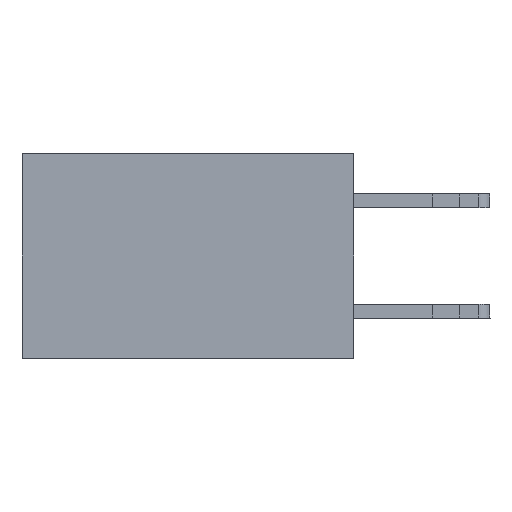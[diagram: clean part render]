
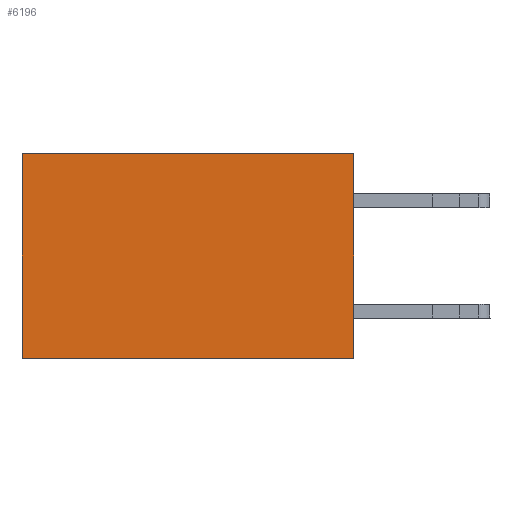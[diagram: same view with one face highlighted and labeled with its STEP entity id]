
A CAD part, left-side view. The second image highlights one B-rep face of the part: STEP entity #6196.
In plain terms, the highlighted planar face has unit normal (-1, 0, 0).
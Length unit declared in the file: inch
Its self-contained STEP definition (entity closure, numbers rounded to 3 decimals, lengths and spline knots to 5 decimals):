
#763 = DIRECTION ( 'NONE',  ( 0., 0., -1. ) ) ;
#1288 = VECTOR ( 'NONE', #11786, 39.37008 ) ;
#1577 = CARTESIAN_POINT ( 'NONE',  ( 0.2875, 0.6, -0.37 ) ) ;
#2237 = CARTESIAN_POINT ( 'NONE',  ( 0.2875, 0., -0.37 ) ) ;
#2305 = VECTOR ( 'NONE', #763, 39.37008 ) ;
#2589 = CARTESIAN_POINT ( 'NONE',  ( 0.2875, 0., 0. ) ) ;
#3010 = LINE ( 'NONE', #9871, #11471 ) ;
#3818 = EDGE_CURVE ( 'NONE', #21166, #11172, #21135, .T. ) ;
#5787 = ORIENTED_EDGE ( 'NONE', *, *, #3818, .T. ) ;
#6196 = ADVANCED_FACE ( 'NONE', ( #18928 ), #8611, .F. ) ;
#6915 = LINE ( 'NONE', #2589, #2305 ) ;
#6938 = CARTESIAN_POINT ( 'NONE',  ( 0.2875, 0., 0. ) ) ;
#7252 = EDGE_CURVE ( 'NONE', #11172, #7948, #3010, .T. ) ;
#7316 = EDGE_CURVE ( 'NONE', #15799, #7948, #10419, .T. ) ;
#7948 = VERTEX_POINT ( 'NONE', #1577 ) ;
#8611 = PLANE ( 'NONE',  #8854 ) ;
#8854 = AXIS2_PLACEMENT_3D ( 'NONE', #6938, #10303, #15276 ) ;
#8898 = CARTESIAN_POINT ( 'NONE',  ( 0.2875, 0., 0. ) ) ;
#9747 = ORIENTED_EDGE ( 'NONE', *, *, #11256, .F. ) ;
#9871 = CARTESIAN_POINT ( 'NONE',  ( 0.2875, 0.6, 0. ) ) ;
#10303 = DIRECTION ( 'NONE',  ( 1., 0., 0. ) ) ;
#10419 = LINE ( 'NONE', #21840, #1288 ) ;
#11172 = VERTEX_POINT ( 'NONE', #12515 ) ;
#11256 = EDGE_CURVE ( 'NONE', #21166, #15799, #6915, .T. ) ;
#11471 = VECTOR ( 'NONE', #21705, 39.37008 ) ;
#11786 = DIRECTION ( 'NONE',  ( 0., 1., 0. ) ) ;
#11814 = CARTESIAN_POINT ( 'NONE',  ( 0.2875, 0., 0. ) ) ;
#12515 = CARTESIAN_POINT ( 'NONE',  ( 0.2875, 0.6, 0. ) ) ;
#14468 = EDGE_LOOP ( 'NONE', ( #21265, #19087, #9747, #5787 ) ) ;
#15276 = DIRECTION ( 'NONE',  ( 0., 0., -1. ) ) ;
#15799 = VERTEX_POINT ( 'NONE', #2237 ) ;
#17311 = DIRECTION ( 'NONE',  ( 0., 1., 0. ) ) ;
#18928 = FACE_OUTER_BOUND ( 'NONE', #14468, .T. ) ;
#19087 = ORIENTED_EDGE ( 'NONE', *, *, #7316, .F. ) ;
#20593 = VECTOR ( 'NONE', #17311, 39.37008 ) ;
#21135 = LINE ( 'NONE', #8898, #20593 ) ;
#21166 = VERTEX_POINT ( 'NONE', #11814 ) ;
#21265 = ORIENTED_EDGE ( 'NONE', *, *, #7252, .T. ) ;
#21705 = DIRECTION ( 'NONE',  ( 0., 0., -1. ) ) ;
#21840 = CARTESIAN_POINT ( 'NONE',  ( 0.2875, 0., -0.37 ) ) ;
